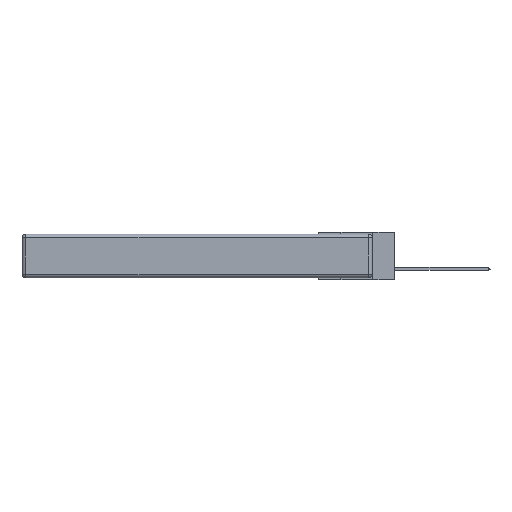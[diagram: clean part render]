
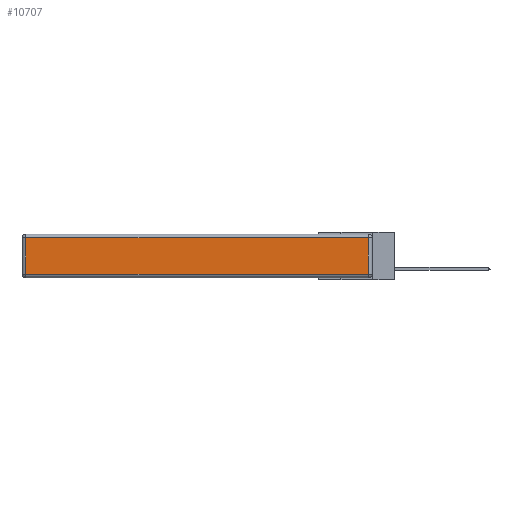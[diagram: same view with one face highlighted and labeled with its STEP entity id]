
A CAD part, left-side view. The second image highlights one B-rep face of the part: STEP entity #10707.
In plain terms, the highlighted planar face has unit normal (-1, 0, 0).
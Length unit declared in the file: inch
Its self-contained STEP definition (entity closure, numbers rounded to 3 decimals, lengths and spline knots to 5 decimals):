
#501 = EDGE_LOOP ( 'NONE', ( #1368, #11105, #9154, #11512 ) ) ;
#526 = CARTESIAN_POINT ( 'NONE',  ( 0., 2.72, -0.03 ) ) ;
#1124 = CARTESIAN_POINT ( 'NONE',  ( 0., 2.72, -0.313 ) ) ;
#1368 = ORIENTED_EDGE ( 'NONE', *, *, #10118, .T. ) ;
#1401 = LINE ( 'NONE', #4729, #9608 ) ;
#2233 = VERTEX_POINT ( 'NONE', #11736 ) ;
#2375 = LINE ( 'NONE', #5870, #8203 ) ;
#2750 = VERTEX_POINT ( 'NONE', #526 ) ;
#3393 = VECTOR ( 'NONE', #9486, 39.37008 ) ;
#3604 = DIRECTION ( 'NONE',  ( -1., 0., 0. ) ) ;
#3669 = CARTESIAN_POINT ( 'NONE',  ( 0., 0.03, -0.03 ) ) ;
#4011 = CARTESIAN_POINT ( 'NONE',  ( 0., 2.72, -0.343 ) ) ;
#4729 = CARTESIAN_POINT ( 'NONE',  ( 0., 0., -0.313 ) ) ;
#5723 = FACE_OUTER_BOUND ( 'NONE', #501, .T. ) ;
#5870 = CARTESIAN_POINT ( 'NONE',  ( 0., 2.75, -0.03 ) ) ;
#5916 = AXIS2_PLACEMENT_3D ( 'NONE', #8842, #3604, #12064 ) ;
#6534 = VERTEX_POINT ( 'NONE', #3669 ) ;
#7489 = LINE ( 'NONE', #10404, #11549 ) ;
#7719 = VERTEX_POINT ( 'NONE', #1124 ) ;
#8203 = VECTOR ( 'NONE', #12583, 39.37008 ) ;
#8510 = PLANE ( 'NONE',  #5916 ) ;
#8842 = CARTESIAN_POINT ( 'NONE',  ( 0., 0., -0.343 ) ) ;
#8911 = EDGE_CURVE ( 'NONE', #2233, #6534, #7489, .T. ) ;
#9154 = ORIENTED_EDGE ( 'NONE', *, *, #13100, .T. ) ;
#9486 = DIRECTION ( 'NONE',  ( 0., 0., -1. ) ) ;
#9608 = VECTOR ( 'NONE', #13359, 39.37008 ) ;
#9634 = LINE ( 'NONE', #4011, #3393 ) ;
#10118 = EDGE_CURVE ( 'NONE', #7719, #2233, #1401, .T. ) ;
#10404 = CARTESIAN_POINT ( 'NONE',  ( 0., 0.03, -0.343 ) ) ;
#10707 = ADVANCED_FACE ( 'NONE', ( #5723 ), #8510, .T. ) ;
#11105 = ORIENTED_EDGE ( 'NONE', *, *, #8911, .T. ) ;
#11119 = EDGE_CURVE ( 'NONE', #2750, #7719, #9634, .T. ) ;
#11512 = ORIENTED_EDGE ( 'NONE', *, *, #11119, .T. ) ;
#11549 = VECTOR ( 'NONE', #13705, 39.37008 ) ;
#11736 = CARTESIAN_POINT ( 'NONE',  ( 0., 0.03, -0.313 ) ) ;
#12064 = DIRECTION ( 'NONE',  ( 0., 0., 1. ) ) ;
#12583 = DIRECTION ( 'NONE',  ( 0., 1., 0. ) ) ;
#13100 = EDGE_CURVE ( 'NONE', #6534, #2750, #2375, .T. ) ;
#13359 = DIRECTION ( 'NONE',  ( 0., -1., 0. ) ) ;
#13705 = DIRECTION ( 'NONE',  ( 0., 0., 1. ) ) ;
